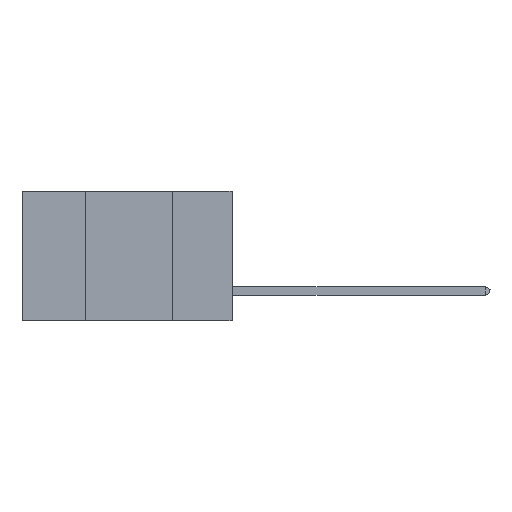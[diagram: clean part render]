
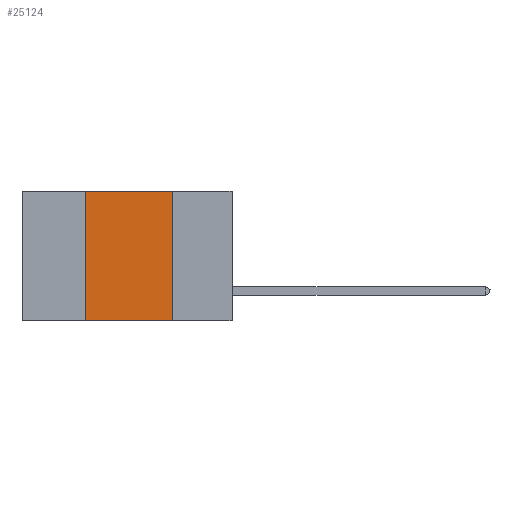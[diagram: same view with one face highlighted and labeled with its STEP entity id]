
A CAD part, left-side view. The second image highlights one B-rep face of the part: STEP entity #25124.
In plain terms, the highlighted planar face has unit normal (-1, 0, 0).
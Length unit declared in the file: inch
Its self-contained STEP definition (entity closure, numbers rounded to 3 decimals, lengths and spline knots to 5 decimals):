
#138 = ORIENTED_EDGE ( 'NONE', *, *, #22444, .F. ) ;
#2332 = VECTOR ( 'NONE', #5045, 39.37008 ) ;
#2425 = VERTEX_POINT ( 'NONE', #11869 ) ;
#2961 = CARTESIAN_POINT ( 'NONE',  ( 0., 0.42, 0. ) ) ;
#3293 = CARTESIAN_POINT ( 'NONE',  ( 0., 0.17, -0.37 ) ) ;
#5045 = DIRECTION ( 'NONE',  ( 0., -1., 0. ) ) ;
#5565 = DIRECTION ( 'NONE',  ( 0., -1., 0. ) ) ;
#6683 = VERTEX_POINT ( 'NONE', #3293 ) ;
#6719 = CARTESIAN_POINT ( 'NONE',  ( 0., 0.17, 0. ) ) ;
#7284 = EDGE_CURVE ( 'NONE', #20696, #6683, #10452, .T. ) ;
#9094 = AXIS2_PLACEMENT_3D ( 'NONE', #32532, #16236, #19324 ) ;
#10452 = LINE ( 'NONE', #24169, #2332 ) ;
#11227 = VECTOR ( 'NONE', #24829, 39.37008 ) ;
#11869 = CARTESIAN_POINT ( 'NONE',  ( 0., 0.17, 0. ) ) ;
#12231 = FACE_OUTER_BOUND ( 'NONE', #25942, .T. ) ;
#13782 = ORIENTED_EDGE ( 'NONE', *, *, #18442, .F. ) ;
#14512 = ORIENTED_EDGE ( 'NONE', *, *, #33733, .F. ) ;
#16236 = DIRECTION ( 'NONE',  ( 1., 0., 0. ) ) ;
#18284 = VERTEX_POINT ( 'NONE', #27864 ) ;
#18442 = EDGE_CURVE ( 'NONE', #20696, #18284, #28374, .T. ) ;
#19164 = CARTESIAN_POINT ( 'NONE',  ( 0., 0.6, 0. ) ) ;
#19324 = DIRECTION ( 'NONE',  ( 0., 0., -1. ) ) ;
#20696 = VERTEX_POINT ( 'NONE', #27144 ) ;
#22444 = EDGE_CURVE ( 'NONE', #2425, #6683, #23613, .T. ) ;
#23613 = LINE ( 'NONE', #6719, #34768 ) ;
#24169 = CARTESIAN_POINT ( 'NONE',  ( 0., 0.6, -0.37 ) ) ;
#24605 = ORIENTED_EDGE ( 'NONE', *, *, #7284, .T. ) ;
#24829 = DIRECTION ( 'NONE',  ( 0., 0., 1. ) ) ;
#24832 = VECTOR ( 'NONE', #5565, 39.37008 ) ;
#25124 = ADVANCED_FACE ( 'NONE', ( #12231 ), #35294, .F. ) ;
#25942 = EDGE_LOOP ( 'NONE', ( #138, #14512, #13782, #24605 ) ) ;
#25978 = DIRECTION ( 'NONE',  ( 0., 0., -1. ) ) ;
#27144 = CARTESIAN_POINT ( 'NONE',  ( 0., 0.42, -0.37 ) ) ;
#27864 = CARTESIAN_POINT ( 'NONE',  ( 0., 0.42, 0. ) ) ;
#28374 = LINE ( 'NONE', #2961, #11227 ) ;
#32123 = LINE ( 'NONE', #19164, #24832 ) ;
#32532 = CARTESIAN_POINT ( 'NONE',  ( 0., 0.6, 0. ) ) ;
#33733 = EDGE_CURVE ( 'NONE', #18284, #2425, #32123, .T. ) ;
#34768 = VECTOR ( 'NONE', #25978, 39.37008 ) ;
#35294 = PLANE ( 'NONE',  #9094 ) ;
